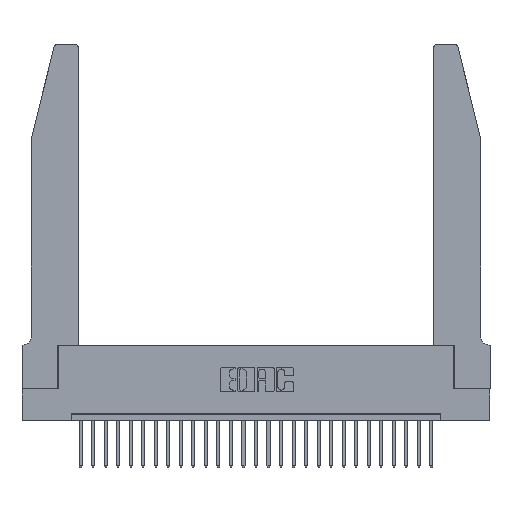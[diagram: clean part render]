
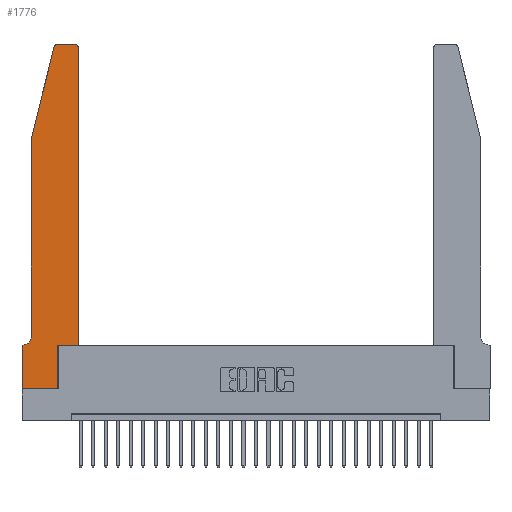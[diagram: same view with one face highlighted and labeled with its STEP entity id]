
A CAD part, top view. The second image highlights one B-rep face of the part: STEP entity #1776.
In plain terms, the highlighted planar face has unit normal (0, 0, 1).
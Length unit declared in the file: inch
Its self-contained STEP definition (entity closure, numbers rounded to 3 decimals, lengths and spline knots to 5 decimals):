
#55 = VERTEX_POINT ( 'NONE', #1942 ) ;
#350 = CARTESIAN_POINT ( 'NONE',  ( 0.4505, 2.72, 0.37 ) ) ;
#375 = DIRECTION ( 'NONE',  ( 1., 0., 0. ) ) ;
#437 = ORIENTED_EDGE ( 'NONE', *, *, #17129, .T. ) ;
#673 = ORIENTED_EDGE ( 'NONE', *, *, #7731, .T. ) ;
#1278 = ORIENTED_EDGE ( 'NONE', *, *, #13262, .T. ) ;
#1439 = DIRECTION ( 'NONE',  ( -1., 0., 0. ) ) ;
#1599 = DIRECTION ( 'NONE',  ( -1., 0., 0. ) ) ;
#1760 = CARTESIAN_POINT ( 'NONE',  ( 0.4205, 2.75, 0.37 ) ) ;
#1776 = ADVANCED_FACE ( 'NONE', ( #13784 ), #6412, .T. ) ;
#1940 = LINE ( 'NONE', #13545, #24516 ) ;
#1942 = CARTESIAN_POINT ( 'NONE',  ( 0.25487, 2.72718, 0.37 ) ) ;
#2007 = EDGE_CURVE ( 'NONE', #16802, #11591, #3803, .T. ) ;
#2045 = CARTESIAN_POINT ( 'NONE',  ( 0.0755, 2., 0.37 ) ) ;
#2329 = AXIS2_PLACEMENT_3D ( 'NONE', #3480, #25598, #16920 ) ;
#2575 = LINE ( 'NONE', #3073, #5283 ) ;
#2667 = VECTOR ( 'NONE', #13457, 39.37008 ) ;
#2779 = ORIENTED_EDGE ( 'NONE', *, *, #25014, .T. ) ;
#3073 = CARTESIAN_POINT ( 'NONE',  ( 0., 0., 0.37 ) ) ;
#3096 = DIRECTION ( 'NONE',  ( -0.239, -0.971, 0. ) ) ;
#3480 = CARTESIAN_POINT ( 'NONE',  ( 0.4205, 2.72, 0.37 ) ) ;
#3803 = LINE ( 'NONE', #7901, #17562 ) ;
#3923 = EDGE_CURVE ( 'NONE', #26337, #55, #26295, .T. ) ;
#4140 = VERTEX_POINT ( 'NONE', #25397 ) ;
#5283 = VECTOR ( 'NONE', #18424, 39.37008 ) ;
#5614 = DIRECTION ( 'NONE',  ( 0., 0., -1. ) ) ;
#5781 = CARTESIAN_POINT ( 'NONE',  ( 0.4505, 0.35, 0.37 ) ) ;
#6240 = VERTEX_POINT ( 'NONE', #22754 ) ;
#6412 = PLANE ( 'NONE',  #26722 ) ;
#6493 = EDGE_LOOP ( 'NONE', ( #2779, #8004, #6933, #13951, #14329, #19622, #14572, #1278, #12214, #437, #673, #23861 ) ) ;
#6828 = EDGE_CURVE ( 'NONE', #16168, #6907, #19382, .T. ) ;
#6907 = VERTEX_POINT ( 'NONE', #1760 ) ;
#6933 = ORIENTED_EDGE ( 'NONE', *, *, #22157, .T. ) ;
#7287 = CARTESIAN_POINT ( 'NONE',  ( 0.0055, 0.35, 0.37 ) ) ;
#7731 = EDGE_CURVE ( 'NONE', #14950, #16168, #22353, .T. ) ;
#7901 = CARTESIAN_POINT ( 'NONE',  ( 0.0755, 0.35, 0.37 ) ) ;
#8004 = ORIENTED_EDGE ( 'NONE', *, *, #3923, .T. ) ;
#8443 = CARTESIAN_POINT ( 'NONE',  ( 0.0755, 2., 0.37 ) ) ;
#8967 = CARTESIAN_POINT ( 'NONE',  ( 0.2605, 2.75, 0.37 ) ) ;
#10339 = CIRCLE ( 'NONE', #12148, 0.07 ) ;
#10620 = VECTOR ( 'NONE', #3096, 39.37008 ) ;
#10850 = DIRECTION ( 'NONE',  ( 0., -1., 0. ) ) ;
#11344 = DIRECTION ( 'NONE',  ( 0., 1., 0. ) ) ;
#11472 = VECTOR ( 'NONE', #10850, 39.37008 ) ;
#11591 = VERTEX_POINT ( 'NONE', #22860 ) ;
#12148 = AXIS2_PLACEMENT_3D ( 'NONE', #21031, #5614, #1439 ) ;
#12214 = ORIENTED_EDGE ( 'NONE', *, *, #12703, .T. ) ;
#12703 = EDGE_CURVE ( 'NONE', #6240, #4140, #1940, .T. ) ;
#12979 = EDGE_CURVE ( 'NONE', #11591, #13454, #2575, .T. ) ;
#13262 = EDGE_CURVE ( 'NONE', #13454, #6240, #14232, .T. ) ;
#13454 = VERTEX_POINT ( 'NONE', #27103 ) ;
#13457 = DIRECTION ( 'NONE',  ( 1., 0., 0. ) ) ;
#13545 = CARTESIAN_POINT ( 'NONE',  ( 0.2865, 0.35, 0.37 ) ) ;
#13784 = FACE_OUTER_BOUND ( 'NONE', #6493, .T. ) ;
#13951 = ORIENTED_EDGE ( 'NONE', *, *, #26475, .T. ) ;
#14232 = LINE ( 'NONE', #23776, #24825 ) ;
#14329 = ORIENTED_EDGE ( 'NONE', *, *, #21069, .T. ) ;
#14572 = ORIENTED_EDGE ( 'NONE', *, *, #12979, .T. ) ;
#14950 = VERTEX_POINT ( 'NONE', #5781 ) ;
#15268 = DIRECTION ( 'NONE',  ( 0., 0., 1. ) ) ;
#15794 = CARTESIAN_POINT ( 'NONE',  ( 0.284, 2.72, 0.37 ) ) ;
#16168 = VERTEX_POINT ( 'NONE', #350 ) ;
#16577 = DIRECTION ( 'NONE',  ( -1., 0., 0. ) ) ;
#16590 = VECTOR ( 'NONE', #27644, 39.37008 ) ;
#16802 = VERTEX_POINT ( 'NONE', #7287 ) ;
#16824 = DIRECTION ( 'NONE',  ( 1., 0., 0. ) ) ;
#16920 = DIRECTION ( 'NONE',  ( 1., 0., 0. ) ) ;
#16921 = CARTESIAN_POINT ( 'NONE',  ( 0.284, 2.75, 0.37 ) ) ;
#17129 = EDGE_CURVE ( 'NONE', #4140, #14950, #19144, .T. ) ;
#17321 = LINE ( 'NONE', #2045, #11472 ) ;
#17562 = VECTOR ( 'NONE', #16577, 39.37008 ) ;
#18035 = VECTOR ( 'NONE', #1599, 39.37008 ) ;
#18080 = DIRECTION ( 'NONE',  ( 0., 0., 1. ) ) ;
#18424 = DIRECTION ( 'NONE',  ( 0., -1., 0. ) ) ;
#19144 = LINE ( 'NONE', #20292, #2667 ) ;
#19382 = CIRCLE ( 'NONE', #2329, 0.03 ) ;
#19511 = VERTEX_POINT ( 'NONE', #24919 ) ;
#19622 = ORIENTED_EDGE ( 'NONE', *, *, #2007, .T. ) ;
#20292 = CARTESIAN_POINT ( 'NONE',  ( 0.4505, 0.35, 0.37 ) ) ;
#20374 = LINE ( 'NONE', #8967, #18035 ) ;
#21031 = CARTESIAN_POINT ( 'NONE',  ( 0.0055, 0.42, 0.37 ) ) ;
#21069 = EDGE_CURVE ( 'NONE', #19511, #16802, #10339, .T. ) ;
#22157 = EDGE_CURVE ( 'NONE', #55, #27401, #22576, .T. ) ;
#22353 = LINE ( 'NONE', #23045, #16590 ) ;
#22576 = LINE ( 'NONE', #22716, #10620 ) ;
#22716 = CARTESIAN_POINT ( 'NONE',  ( 0.0755, 2., 0.37 ) ) ;
#22754 = CARTESIAN_POINT ( 'NONE',  ( 0.2865, 0., 0.37 ) ) ;
#22860 = CARTESIAN_POINT ( 'NONE',  ( 0., 0.35, 0.37 ) ) ;
#23045 = CARTESIAN_POINT ( 'NONE',  ( 0.4505, 0.35, 0.37 ) ) ;
#23776 = CARTESIAN_POINT ( 'NONE',  ( 0., 0., 0.37 ) ) ;
#23861 = ORIENTED_EDGE ( 'NONE', *, *, #6828, .T. ) ;
#24516 = VECTOR ( 'NONE', #11344, 39.37008 ) ;
#24825 = VECTOR ( 'NONE', #16824, 39.37008 ) ;
#24919 = CARTESIAN_POINT ( 'NONE',  ( 0.0755, 0.42, 0.37 ) ) ;
#25014 = EDGE_CURVE ( 'NONE', #6907, #26337, #20374, .T. ) ;
#25397 = CARTESIAN_POINT ( 'NONE',  ( 0.2865, 0.35, 0.37 ) ) ;
#25598 = DIRECTION ( 'NONE',  ( 0., 0., 1. ) ) ;
#25790 = AXIS2_PLACEMENT_3D ( 'NONE', #15794, #18080, #26477 ) ;
#26148 = CARTESIAN_POINT ( 'NONE',  ( 0., 0.35, 0.37 ) ) ;
#26295 = CIRCLE ( 'NONE', #25790, 0.03 ) ;
#26337 = VERTEX_POINT ( 'NONE', #16921 ) ;
#26475 = EDGE_CURVE ( 'NONE', #27401, #19511, #17321, .T. ) ;
#26477 = DIRECTION ( 'NONE',  ( 1., 0., 0. ) ) ;
#26722 = AXIS2_PLACEMENT_3D ( 'NONE', #26148, #15268, #375 ) ;
#27103 = CARTESIAN_POINT ( 'NONE',  ( 0., 0., 0.37 ) ) ;
#27401 = VERTEX_POINT ( 'NONE', #8443 ) ;
#27644 = DIRECTION ( 'NONE',  ( 0., 1., 0. ) ) ;
